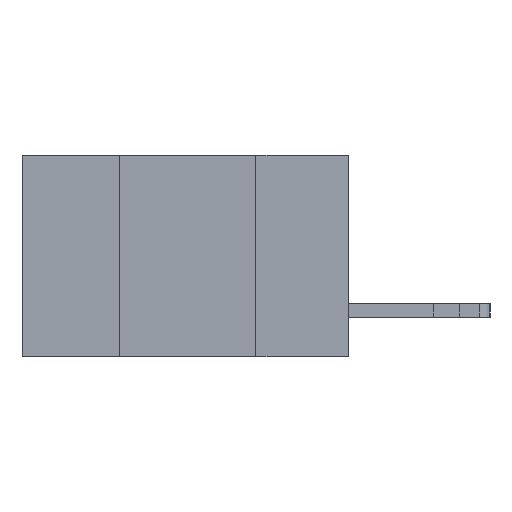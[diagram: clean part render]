
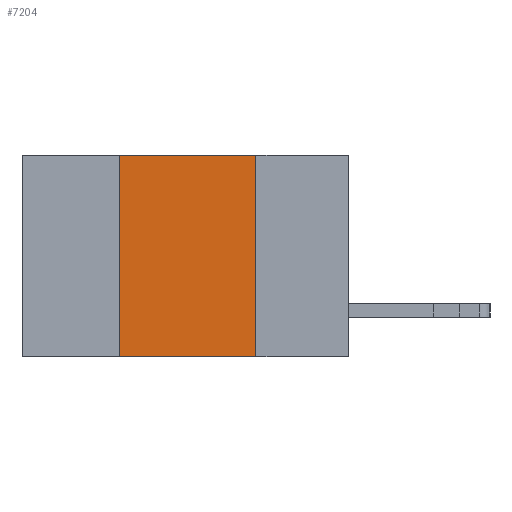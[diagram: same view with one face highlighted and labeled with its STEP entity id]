
A CAD part, left-side view. The second image highlights one B-rep face of the part: STEP entity #7204.
In plain terms, the highlighted planar face has unit normal (-1, 0, 0).
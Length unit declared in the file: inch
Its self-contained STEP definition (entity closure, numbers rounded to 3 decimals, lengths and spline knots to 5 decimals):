
#140 = VECTOR ( 'NONE', #3602, 39.37008 ) ;
#238 = EDGE_CURVE ( 'NONE', #7275, #2899, #2693, .T. ) ;
#681 = VECTOR ( 'NONE', #4166, 39.37008 ) ;
#1283 = FACE_OUTER_BOUND ( 'NONE', #8796, .T. ) ;
#1604 = CARTESIAN_POINT ( 'NONE',  ( 0., 0.17, -0.37 ) ) ;
#2369 = ORIENTED_EDGE ( 'NONE', *, *, #4115, .F. ) ;
#2404 = DIRECTION ( 'NONE',  ( 0., 0., -1. ) ) ;
#2693 = LINE ( 'NONE', #7344, #4319 ) ;
#2899 = VERTEX_POINT ( 'NONE', #8147 ) ;
#3602 = DIRECTION ( 'NONE',  ( 0., -1., 0. ) ) ;
#4009 = ORIENTED_EDGE ( 'NONE', *, *, #6742, .F. ) ;
#4090 = CARTESIAN_POINT ( 'NONE',  ( 0., 0.42, 0. ) ) ;
#4115 = EDGE_CURVE ( 'NONE', #6912, #7275, #7896, .T. ) ;
#4166 = DIRECTION ( 'NONE',  ( 0., 0., -1. ) ) ;
#4253 = ORIENTED_EDGE ( 'NONE', *, *, #238, .F. ) ;
#4319 = VECTOR ( 'NONE', #8808, 39.37008 ) ;
#4580 = LINE ( 'NONE', #8506, #140 ) ;
#5593 = CARTESIAN_POINT ( 'NONE',  ( 0., 0.6, 0. ) ) ;
#5666 = VECTOR ( 'NONE', #6610, 39.37008 ) ;
#5685 = CARTESIAN_POINT ( 'NONE',  ( 0., 0.17, -0.37 ) ) ;
#6430 = PLANE ( 'NONE',  #10363 ) ;
#6610 = DIRECTION ( 'NONE',  ( 0., 0., 1. ) ) ;
#6678 = ORIENTED_EDGE ( 'NONE', *, *, #9166, .T. ) ;
#6742 = EDGE_CURVE ( 'NONE', #2899, #8897, #7471, .T. ) ;
#6808 = CARTESIAN_POINT ( 'NONE',  ( 0., 0.42, -0.37 ) ) ;
#6912 = VERTEX_POINT ( 'NONE', #6808 ) ;
#7186 = CARTESIAN_POINT ( 'NONE',  ( 0., 0.42, -0.37 ) ) ;
#7204 = ADVANCED_FACE ( 'NONE', ( #1283 ), #6430, .F. ) ;
#7275 = VERTEX_POINT ( 'NONE', #4090 ) ;
#7291 = DIRECTION ( 'NONE',  ( 1., 0., 0. ) ) ;
#7344 = CARTESIAN_POINT ( 'NONE',  ( 0., 0.6, 0. ) ) ;
#7471 = LINE ( 'NONE', #1604, #681 ) ;
#7896 = LINE ( 'NONE', #7186, #5666 ) ;
#8147 = CARTESIAN_POINT ( 'NONE',  ( 0., 0.17, 0. ) ) ;
#8506 = CARTESIAN_POINT ( 'NONE',  ( 0., 0.6, -0.37 ) ) ;
#8796 = EDGE_LOOP ( 'NONE', ( #4009, #4253, #2369, #6678 ) ) ;
#8808 = DIRECTION ( 'NONE',  ( 0., -1., 0. ) ) ;
#8897 = VERTEX_POINT ( 'NONE', #5685 ) ;
#9166 = EDGE_CURVE ( 'NONE', #6912, #8897, #4580, .T. ) ;
#10363 = AXIS2_PLACEMENT_3D ( 'NONE', #5593, #7291, #2404 ) ;
